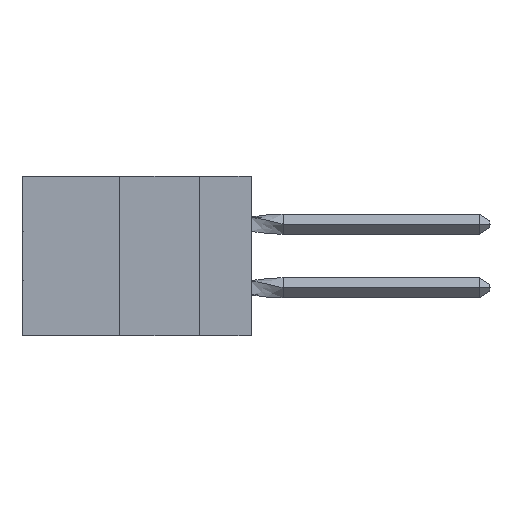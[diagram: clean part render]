
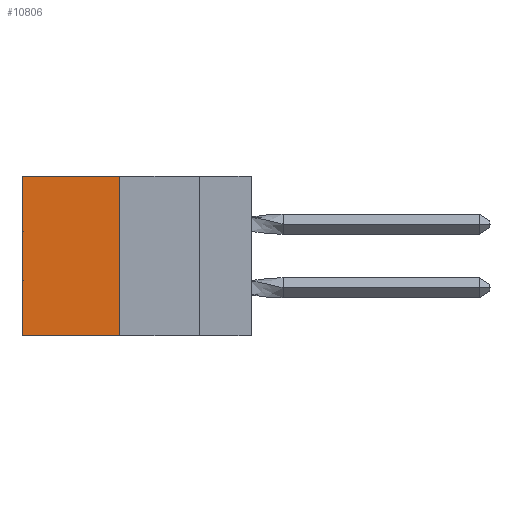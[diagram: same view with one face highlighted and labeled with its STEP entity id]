
A CAD part, left-side view. The second image highlights one B-rep face of the part: STEP entity #10806.
In plain terms, the highlighted planar face has unit normal (-1, 0, 0).
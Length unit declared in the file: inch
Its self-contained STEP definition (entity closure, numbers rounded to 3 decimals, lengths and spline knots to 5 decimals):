
#206 = CARTESIAN_POINT ( 'NONE',  ( 0.305, 0.72, -0.5 ) ) ;
#1591 = ORIENTED_EDGE ( 'NONE', *, *, #3499, .T. ) ;
#3499 = EDGE_CURVE ( 'NONE', #7802, #22343, #39013, .T. ) ;
#5957 = ORIENTED_EDGE ( 'NONE', *, *, #21194, .F. ) ;
#7802 = VERTEX_POINT ( 'NONE', #10036 ) ;
#7818 = DIRECTION ( 'NONE',  ( 0., 0., -1. ) ) ;
#9435 = VECTOR ( 'NONE', #15174, 39.37008 ) ;
#10036 = CARTESIAN_POINT ( 'NONE',  ( 0.305, 0.413, 0. ) ) ;
#10806 = ADVANCED_FACE ( 'NONE', ( #30913 ), #30333, .F. ) ;
#13819 = CARTESIAN_POINT ( 'NONE',  ( 0.305, 0.413, -0.5 ) ) ;
#15174 = DIRECTION ( 'NONE',  ( 0., 1., 0. ) ) ;
#16765 = EDGE_LOOP ( 'NONE', ( #39295, #5957, #20965, #1591 ) ) ;
#18014 = AXIS2_PLACEMENT_3D ( 'NONE', #33405, #39679, #7818 ) ;
#19588 = CARTESIAN_POINT ( 'NONE',  ( 0.305, 0.413, -0.5 ) ) ;
#19673 = EDGE_CURVE ( 'NONE', #22343, #26167, #24971, .T. ) ;
#20965 = ORIENTED_EDGE ( 'NONE', *, *, #41420, .F. ) ;
#21194 = EDGE_CURVE ( 'NONE', #25175, #26167, #35370, .T. ) ;
#22343 = VERTEX_POINT ( 'NONE', #26773 ) ;
#22797 = DIRECTION ( 'NONE',  ( 0., 1., 0. ) ) ;
#24971 = LINE ( 'NONE', #30522, #33535 ) ;
#25175 = VERTEX_POINT ( 'NONE', #13819 ) ;
#26167 = VERTEX_POINT ( 'NONE', #206 ) ;
#26773 = CARTESIAN_POINT ( 'NONE',  ( 0.305, 0.72, 0. ) ) ;
#28361 = CARTESIAN_POINT ( 'NONE',  ( 0.305, 0.413, 0. ) ) ;
#29887 = VECTOR ( 'NONE', #22797, 39.37008 ) ;
#30333 = PLANE ( 'NONE',  #18014 ) ;
#30522 = CARTESIAN_POINT ( 'NONE',  ( 0.305, 0.72, -0.5 ) ) ;
#30636 = CARTESIAN_POINT ( 'NONE',  ( 0.305, 0.413, -0.5 ) ) ;
#30913 = FACE_OUTER_BOUND ( 'NONE', #16765, .T. ) ;
#33405 = CARTESIAN_POINT ( 'NONE',  ( 0.305, 0.413, -0.5 ) ) ;
#33535 = VECTOR ( 'NONE', #36966, 39.37008 ) ;
#35370 = LINE ( 'NONE', #19588, #29887 ) ;
#36966 = DIRECTION ( 'NONE',  ( 0., 0., -1. ) ) ;
#37912 = DIRECTION ( 'NONE',  ( 0., 0., -1. ) ) ;
#39013 = LINE ( 'NONE', #28361, #9435 ) ;
#39295 = ORIENTED_EDGE ( 'NONE', *, *, #19673, .T. ) ;
#39679 = DIRECTION ( 'NONE',  ( 1., 0., 0. ) ) ;
#40939 = VECTOR ( 'NONE', #37912, 39.37008 ) ;
#41420 = EDGE_CURVE ( 'NONE', #7802, #25175, #41428, .T. ) ;
#41428 = LINE ( 'NONE', #30636, #40939 ) ;
